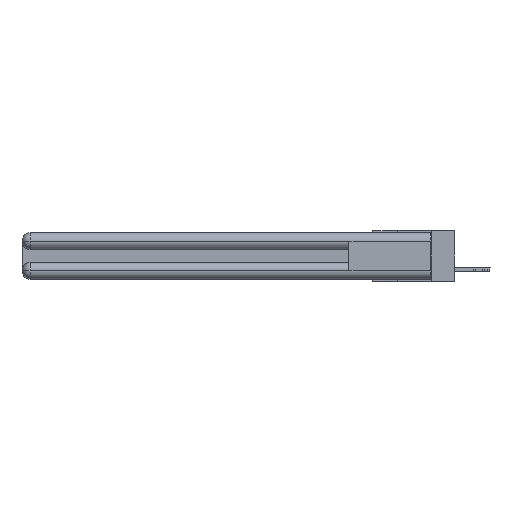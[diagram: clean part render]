
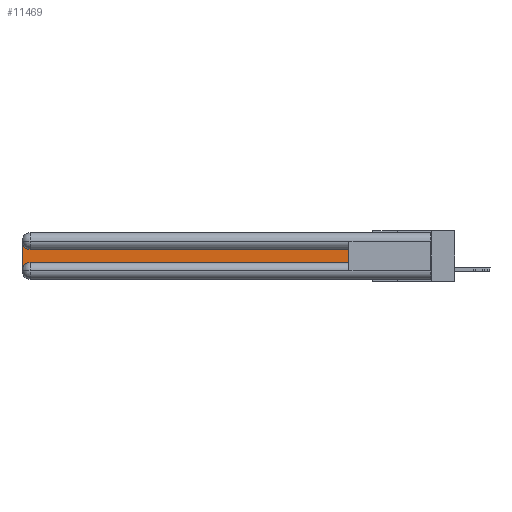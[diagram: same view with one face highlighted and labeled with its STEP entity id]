
A CAD part, left-side view. The second image highlights one B-rep face of the part: STEP entity #11469.
In plain terms, the highlighted planar face has unit normal (-1, 0, 0).
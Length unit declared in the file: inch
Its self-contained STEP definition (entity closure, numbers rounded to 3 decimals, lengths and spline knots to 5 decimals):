
#602 = LINE ( 'NONE', #4121, #20964 ) ;
#630 = EDGE_CURVE ( 'NONE', #15650, #4652, #18664, .T. ) ;
#1970 = VERTEX_POINT ( 'NONE', #15239 ) ;
#2765 = DIRECTION ( 'NONE',  ( 1., 0., 0. ) ) ;
#3708 = CARTESIAN_POINT ( 'NONE',  ( 0.075, 2.94, -0.1225 ) ) ;
#3999 = DIRECTION ( 'NONE',  ( 0., -1., 0. ) ) ;
#4121 = CARTESIAN_POINT ( 'NONE',  ( 0.075, 0.6, -0.2175 ) ) ;
#4350 = LINE ( 'NONE', #16329, #34411 ) ;
#4652 = VERTEX_POINT ( 'NONE', #21164 ) ;
#5360 = VERTEX_POINT ( 'NONE', #31644 ) ;
#7245 = EDGE_LOOP ( 'NONE', ( #13499, #25540, #24411, #26261, #21876, #29178 ) ) ;
#7730 = VECTOR ( 'NONE', #20290, 39.37008 ) ;
#8558 = EDGE_CURVE ( 'NONE', #33195, #32119, #26318, .T. ) ;
#10906 = CARTESIAN_POINT ( 'NONE',  ( 0.075, 2.94, -0.2775 ) ) ;
#11469 = ADVANCED_FACE ( 'NONE', ( #18220 ), #22609, .F. ) ;
#12022 = CARTESIAN_POINT ( 'NONE',  ( 0.075, 0.6, -0.1225 ) ) ;
#12486 = CARTESIAN_POINT ( 'NONE',  ( 0.075, 2.94, -0.0625 ) ) ;
#12707 = DIRECTION ( 'NONE',  ( 1., 0., 0. ) ) ;
#13334 = VECTOR ( 'NONE', #3999, 39.37008 ) ;
#13499 = ORIENTED_EDGE ( 'NONE', *, *, #21951, .T. ) ;
#14677 = CARTESIAN_POINT ( 'NONE',  ( 0.075, 3., -0.1225 ) ) ;
#15239 = CARTESIAN_POINT ( 'NONE',  ( 0.075, 0.6, -0.2175 ) ) ;
#15650 = VERTEX_POINT ( 'NONE', #21602 ) ;
#16329 = CARTESIAN_POINT ( 'NONE',  ( 0.075, 3., -0.2175 ) ) ;
#17614 = EDGE_CURVE ( 'NONE', #1970, #5360, #602, .T. ) ;
#18220 = FACE_OUTER_BOUND ( 'NONE', #7245, .T. ) ;
#18664 = CIRCLE ( 'NONE', #26766, 0.06 ) ;
#19023 = DIRECTION ( 'NONE',  ( 0., 0., -1. ) ) ;
#19173 = AXIS2_PLACEMENT_3D ( 'NONE', #14677, #25881, #20970 ) ;
#19614 = LINE ( 'NONE', #27874, #13334 ) ;
#19876 = EDGE_CURVE ( 'NONE', #4652, #1970, #19614, .T. ) ;
#19967 = AXIS2_PLACEMENT_3D ( 'NONE', #12486, #12707, #34013 ) ;
#20290 = DIRECTION ( 'NONE',  ( 0., 1., 0. ) ) ;
#20964 = VECTOR ( 'NONE', #33621, 39.37008 ) ;
#20970 = DIRECTION ( 'NONE',  ( 0., 0., -1. ) ) ;
#21164 = CARTESIAN_POINT ( 'NONE',  ( 0.075, 2.94, -0.2175 ) ) ;
#21602 = CARTESIAN_POINT ( 'NONE',  ( 0.075, 3., -0.2775 ) ) ;
#21876 = ORIENTED_EDGE ( 'NONE', *, *, #19876, .T. ) ;
#21951 = EDGE_CURVE ( 'NONE', #5360, #33195, #33244, .T. ) ;
#22609 = PLANE ( 'NONE',  #19173 ) ;
#24411 = ORIENTED_EDGE ( 'NONE', *, *, #32516, .T. ) ;
#25540 = ORIENTED_EDGE ( 'NONE', *, *, #8558, .T. ) ;
#25881 = DIRECTION ( 'NONE',  ( 1., 0., 0. ) ) ;
#26261 = ORIENTED_EDGE ( 'NONE', *, *, #630, .T. ) ;
#26318 = CIRCLE ( 'NONE', #19967, 0.06 ) ;
#26766 = AXIS2_PLACEMENT_3D ( 'NONE', #10906, #2765, #29233 ) ;
#27874 = CARTESIAN_POINT ( 'NONE',  ( 0.075, 0.6, -0.2175 ) ) ;
#29178 = ORIENTED_EDGE ( 'NONE', *, *, #17614, .T. ) ;
#29233 = DIRECTION ( 'NONE',  ( 0., 0., -1. ) ) ;
#31633 = CARTESIAN_POINT ( 'NONE',  ( 0.075, 3., -0.0625 ) ) ;
#31644 = CARTESIAN_POINT ( 'NONE',  ( 0.075, 0.6, -0.1225 ) ) ;
#32119 = VERTEX_POINT ( 'NONE', #31633 ) ;
#32516 = EDGE_CURVE ( 'NONE', #32119, #15650, #4350, .T. ) ;
#33195 = VERTEX_POINT ( 'NONE', #3708 ) ;
#33244 = LINE ( 'NONE', #12022, #7730 ) ;
#33621 = DIRECTION ( 'NONE',  ( 0., 0., 1. ) ) ;
#34013 = DIRECTION ( 'NONE',  ( 0., 0., -1. ) ) ;
#34411 = VECTOR ( 'NONE', #19023, 39.37008 ) ;
